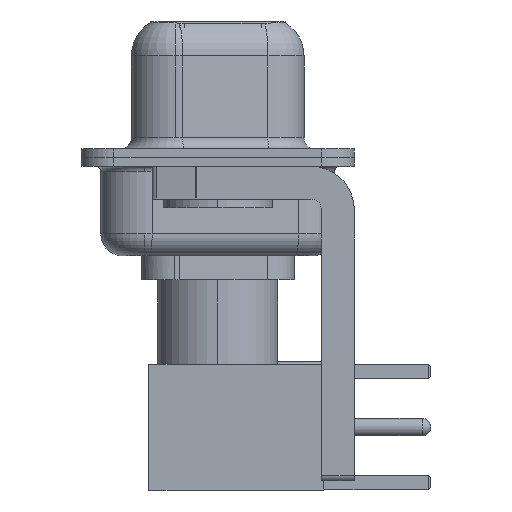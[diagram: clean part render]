
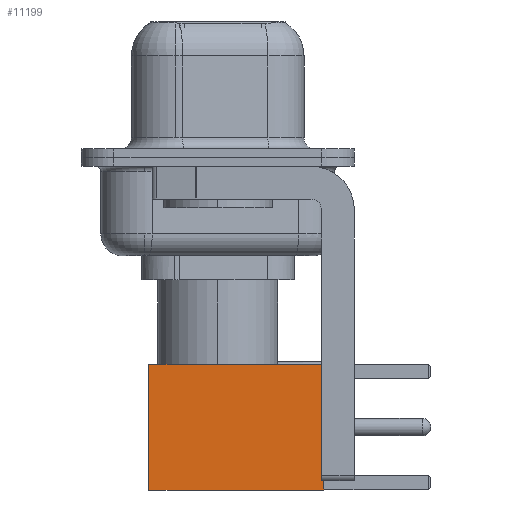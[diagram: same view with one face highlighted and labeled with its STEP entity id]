
A CAD part, left-side view. The second image highlights one B-rep face of the part: STEP entity #11199.
In plain terms, the highlighted face is planar.
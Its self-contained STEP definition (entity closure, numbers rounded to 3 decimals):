
#126 = ORIENTED_EDGE ( 'NONE', *, *, #22743, .T. ) ;
#1321 = ORIENTED_EDGE ( 'NONE', *, *, #17168, .F. ) ;
#1715 = DIRECTION ( 'NONE',  ( 0., 0., -1. ) ) ;
#2392 = LINE ( 'NONE', #24759, #15783 ) ;
#3997 = LINE ( 'NONE', #17531, #20096 ) ;
#4460 = DIRECTION ( 'NONE',  ( 0., 1., 0. ) ) ;
#4543 = CARTESIAN_POINT ( 'NONE',  ( 2.875, 2.875, 8. ) ) ;
#4718 = DIRECTION ( 'NONE',  ( 0., 0., 1. ) ) ;
#5432 = DIRECTION ( 'NONE',  ( -1., 0., 0. ) ) ;
#9267 = DIRECTION ( 'NONE',  ( -1., 0., 0. ) ) ;
#9775 = VECTOR ( 'NONE', #5432, 1000. ) ;
#11177 = ORIENTED_EDGE ( 'NONE', *, *, #14619, .F. ) ;
#11199 = ADVANCED_FACE ( 'NONE', ( #14738 ), #21119, .T. ) ;
#11294 = LINE ( 'NONE', #13470, #15027 ) ;
#11496 = CARTESIAN_POINT ( 'NONE',  ( -2.875, 2.875, 8. ) ) ;
#11522 = CARTESIAN_POINT ( 'NONE',  ( 0., 2.875, 0. ) ) ;
#13470 = CARTESIAN_POINT ( 'NONE',  ( 0., 2.875, 8. ) ) ;
#14421 = VERTEX_POINT ( 'NONE', #24355 ) ;
#14619 = EDGE_CURVE ( 'NONE', #21589, #15530, #2392, .T. ) ;
#14738 = FACE_OUTER_BOUND ( 'NONE', #24219, .T. ) ;
#14955 = DIRECTION ( 'NONE',  ( 0., 0., -1. ) ) ;
#15027 = VECTOR ( 'NONE', #9267, 1000. ) ;
#15478 = EDGE_CURVE ( 'NONE', #14421, #15530, #21847, .T. ) ;
#15530 = VERTEX_POINT ( 'NONE', #21109 ) ;
#15783 = VECTOR ( 'NONE', #14955, 1000. ) ;
#17168 = EDGE_CURVE ( 'NONE', #23774, #21589, #11294, .T. ) ;
#17531 = CARTESIAN_POINT ( 'NONE',  ( 2.875, 2.875, 0. ) ) ;
#20096 = VECTOR ( 'NONE', #1715, 1000. ) ;
#21109 = CARTESIAN_POINT ( 'NONE',  ( -2.875, 2.875, 0. ) ) ;
#21119 = PLANE ( 'NONE',  #23518 ) ;
#21589 = VERTEX_POINT ( 'NONE', #11496 ) ;
#21847 = LINE ( 'NONE', #11522, #9775 ) ;
#22092 = ORIENTED_EDGE ( 'NONE', *, *, #15478, .T. ) ;
#22743 = EDGE_CURVE ( 'NONE', #23774, #14421, #3997, .T. ) ;
#23424 = CARTESIAN_POINT ( 'NONE',  ( 2.875, 2.875, 0. ) ) ;
#23518 = AXIS2_PLACEMENT_3D ( 'NONE', #23424, #4460, #4718 ) ;
#23774 = VERTEX_POINT ( 'NONE', #4543 ) ;
#24219 = EDGE_LOOP ( 'NONE', ( #126, #22092, #11177, #1321 ) ) ;
#24355 = CARTESIAN_POINT ( 'NONE',  ( 2.875, 2.875, 0. ) ) ;
#24759 = CARTESIAN_POINT ( 'NONE',  ( -2.875, 2.875, 0. ) ) ;
